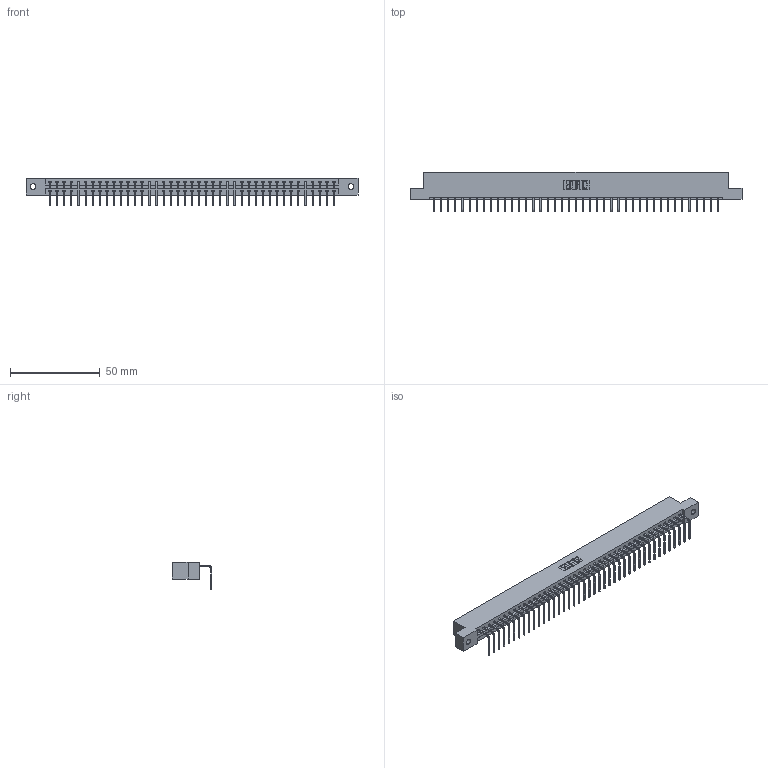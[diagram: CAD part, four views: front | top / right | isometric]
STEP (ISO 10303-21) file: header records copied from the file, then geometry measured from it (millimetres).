
FILE_DESCRIPTION (( 'STEP AP203' ), '1' );
FILE_NAME ('387-041-558-102.STEP', '2019-10-07T21:34:20', ( '' ), ( '' ), 'SwSTEP 2.0', 'SolidWorks 2016', '' );
FILE_SCHEMA (( 'CONFIG_CONTROL_DESIGN' ));
Length unit declared in the file: inch
Products named in the file (3): 387-041-558-102; 345-292-001_558 Tail - 2; 337 Part_Flush Mounting Lugs - 0.128 Dia
Assembly tree (42 placements, depth 2):
  387-041-558-102
    337 Part_Flush Mounting Lugs - 0.128 Dia
    345-292-001_558 Tail - 2  x41
Bounding box: 185.47 x 22.17 x 15.37 mm (x, y, z)
Volume: 19364 mm3; surface area: 20573.6 mm2
Topology: 42 solids, 42 shells, 2738 faces, 8265 edges, 5454 vertices
Faces by surface type: plane 2038, cylinder 700
Entity records: 30693 total; most frequent: CARTESIAN_POINT 5353, ORIENTED_EDGE 5330, DIRECTION 4507, EDGE_CURVE 2665, LINE 2537, VECTOR 2537, VERTEX_POINT 1774, AXIS2_PLACEMENT_3D 985
